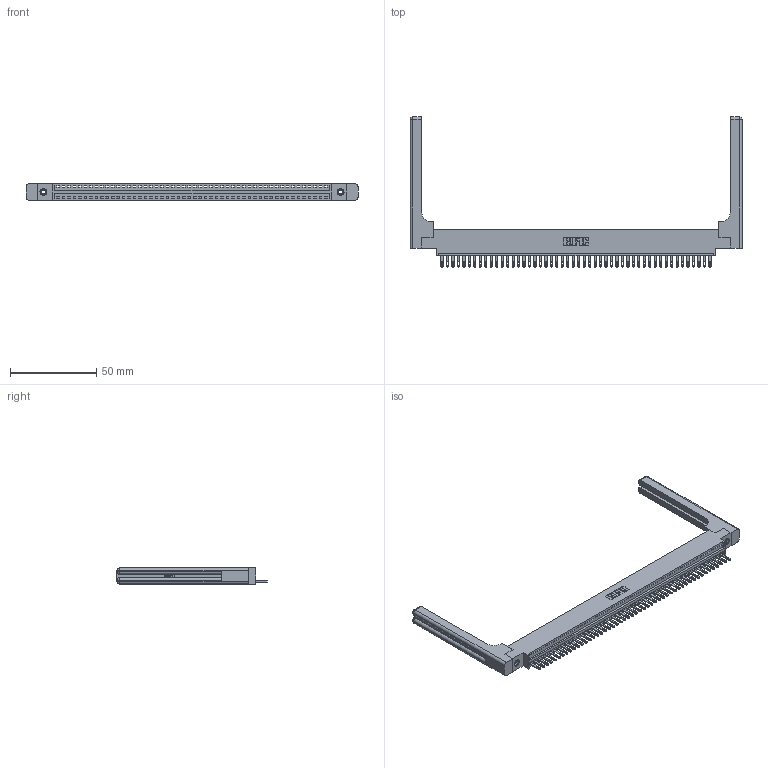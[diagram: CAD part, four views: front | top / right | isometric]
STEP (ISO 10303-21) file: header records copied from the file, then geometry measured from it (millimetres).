
FILE_DESCRIPTION (( 'STEP AP203' ), '1' );
FILE_NAME ('346-050-500-658.STEP', '2022-05-10T02:36:56', ( '' ), ( '' ), 'SwSTEP 2.0', 'SolidWorks 2020', '' );
FILE_SCHEMA (( 'CONFIG_CONTROL_DESIGN' ));
Length unit declared in the file: inch
Products named in the file (5): 346 Part_0.170 Offset - 0.156 Dia-TH; 345-292-001_345-293-100; 346-220-058_345-220-058; 345-250-001_345-250-001-102; 346-050-500-658
Assembly tree (55 placements, depth 2):
  346-050-500-658
    346 Part_0.170 Offset - 0.156 Dia-TH
    345-292-001_345-293-100  x50
    345-250-001_345-250-001-102  x2
    346-220-058_345-220-058  x2
Bounding box: 192.81 x 87.12 x 9.4 mm (x, y, z)
Volume: 25888.1 mm3; surface area: 28524.7 mm2
Topology: 55 solids, 55 shells, 3096 faces, 9443 edges, 6274 vertices
Faces by surface type: plane 1942, cylinder 1094, bspline 36, cone 12, sphere 8, torus 4
Entity records: 35614 total; most frequent: CARTESIAN_POINT 7085, ORIENTED_EDGE 5864, DIRECTION 5172, EDGE_CURVE 2932, VECTOR 2504, LINE 2504, VERTEX_POINT 1946, AXIS2_PLACEMENT_3D 1334
